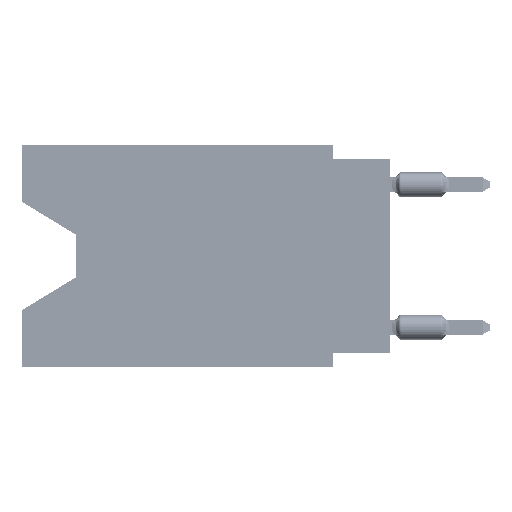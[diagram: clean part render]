
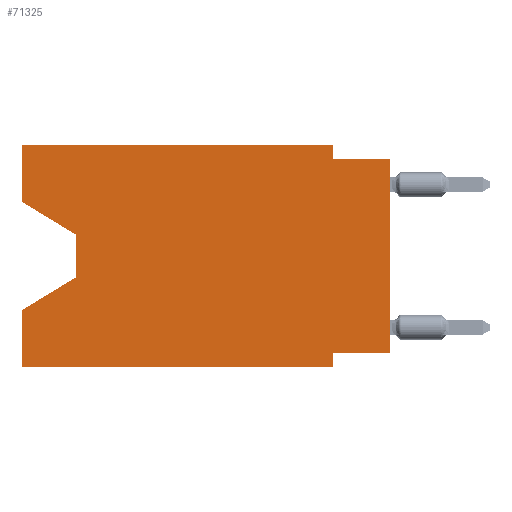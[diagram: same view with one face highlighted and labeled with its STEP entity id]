
A CAD part, left-side view. The second image highlights one B-rep face of the part: STEP entity #71325.
In plain terms, the highlighted planar face has unit normal (-1, 0, 0).
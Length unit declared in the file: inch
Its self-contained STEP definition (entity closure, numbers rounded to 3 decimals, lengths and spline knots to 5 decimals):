
#85 = CARTESIAN_POINT ( 'NONE',  ( 0., 0.645, 0. ) ) ;
#205 = CARTESIAN_POINT ( 'NONE',  ( 0., 0., 0. ) ) ;
#1108 = LINE ( 'NONE', #30797, #12926 ) ;
#4116 = EDGE_CURVE ( 'NONE', #9246, #67004, #49657, .T. ) ;
#4400 = EDGE_CURVE ( 'NONE', #48694, #24172, #54074, .T. ) ;
#4721 = ORIENTED_EDGE ( 'NONE', *, *, #23242, .F. ) ;
#5830 = CARTESIAN_POINT ( 'NONE',  ( 0., 0.645, -0.39 ) ) ;
#6450 = VECTOR ( 'NONE', #14433, 39.37008 ) ;
#6566 = VECTOR ( 'NONE', #40404, 39.37008 ) ;
#7133 = EDGE_CURVE ( 'NONE', #48694, #78525, #32270, .T. ) ;
#8567 = DIRECTION ( 'NONE',  ( 1., 0., 0. ) ) ;
#9246 = VERTEX_POINT ( 'NONE', #50335 ) ;
#9248 = LINE ( 'NONE', #72170, #31322 ) ;
#9652 = DIRECTION ( 'NONE',  ( 0., -0.855, -0.519 ) ) ;
#9934 = CARTESIAN_POINT ( 'NONE',  ( 0., 0.645, 0. ) ) ;
#10221 = CARTESIAN_POINT ( 'NONE',  ( 0., 0., -0.365 ) ) ;
#10315 = CARTESIAN_POINT ( 'NONE',  ( 0., 0.55, -0.158 ) ) ;
#10739 = VECTOR ( 'NONE', #42714, 39.37008 ) ;
#11453 = CARTESIAN_POINT ( 'NONE',  ( 0., 0.55, -0.158 ) ) ;
#12619 = ORIENTED_EDGE ( 'NONE', *, *, #4400, .F. ) ;
#12926 = VECTOR ( 'NONE', #68530, 39.37008 ) ;
#12966 = VERTEX_POINT ( 'NONE', #50551 ) ;
#13065 = EDGE_CURVE ( 'NONE', #71305, #78525, #18894, .T. ) ;
#14186 = ORIENTED_EDGE ( 'NONE', *, *, #52523, .T. ) ;
#14433 = DIRECTION ( 'NONE',  ( 0., 0., -1. ) ) ;
#15061 = ORIENTED_EDGE ( 'NONE', *, *, #55617, .T. ) ;
#16561 = VERTEX_POINT ( 'NONE', #10315 ) ;
#16594 = ORIENTED_EDGE ( 'NONE', *, *, #4116, .T. ) ;
#18894 = LINE ( 'NONE', #74912, #41798 ) ;
#19269 = DIRECTION ( 'NONE',  ( 0., 0., 1. ) ) ;
#19307 = VECTOR ( 'NONE', #73506, 39.37008 ) ;
#20121 = CARTESIAN_POINT ( 'NONE',  ( 0., 0.1, -0.39 ) ) ;
#21328 = CARTESIAN_POINT ( 'NONE',  ( 0., 0.1, -0.39 ) ) ;
#22410 = CARTESIAN_POINT ( 'NONE',  ( 0., 0.55, -0.232 ) ) ;
#22863 = CARTESIAN_POINT ( 'NONE',  ( 0., 0.645, -0.28975 ) ) ;
#23242 = EDGE_CURVE ( 'NONE', #24172, #67004, #46086, .T. ) ;
#24172 = VERTEX_POINT ( 'NONE', #58494 ) ;
#24850 = DIRECTION ( 'NONE',  ( 0., -1., 0. ) ) ;
#25305 = EDGE_CURVE ( 'NONE', #12966, #71305, #51599, .T. ) ;
#25319 = VECTOR ( 'NONE', #71940, 39.37008 ) ;
#29825 = VERTEX_POINT ( 'NONE', #40304 ) ;
#30617 = DIRECTION ( 'NONE',  ( 0., -1., 0. ) ) ;
#30797 = CARTESIAN_POINT ( 'NONE',  ( 0., 0.645, 0. ) ) ;
#31322 = VECTOR ( 'NONE', #9652, 39.37008 ) ;
#32270 = LINE ( 'NONE', #205, #74461 ) ;
#33681 = ORIENTED_EDGE ( 'NONE', *, *, #46680, .F. ) ;
#35033 = ORIENTED_EDGE ( 'NONE', *, *, #13065, .F. ) ;
#36433 = EDGE_CURVE ( 'NONE', #29825, #74711, #1108, .T. ) ;
#36576 = CARTESIAN_POINT ( 'NONE',  ( 0., 0.55, -0.232 ) ) ;
#37591 = CARTESIAN_POINT ( 'NONE',  ( 0., 0.645, 0. ) ) ;
#38622 = PLANE ( 'NONE',  #73836 ) ;
#39627 = VERTEX_POINT ( 'NONE', #22863 ) ;
#40304 = CARTESIAN_POINT ( 'NONE',  ( 0., 0.645, -0.10025 ) ) ;
#40404 = DIRECTION ( 'NONE',  ( 0., 0., 1. ) ) ;
#41792 = EDGE_CURVE ( 'NONE', #16561, #75496, #66691, .T. ) ;
#41798 = VECTOR ( 'NONE', #56646, 39.37008 ) ;
#42714 = DIRECTION ( 'NONE',  ( 0., 0., -1. ) ) ;
#44713 = FACE_OUTER_BOUND ( 'NONE', #45901, .T. ) ;
#45074 = VECTOR ( 'NONE', #24850, 39.37008 ) ;
#45112 = CARTESIAN_POINT ( 'NONE',  ( 0., 0.1, -0.025 ) ) ;
#45301 = ORIENTED_EDGE ( 'NONE', *, *, #36433, .F. ) ;
#45901 = EDGE_LOOP ( 'NONE', ( #15061, #56737, #14186, #62089, #16594, #4721, #12619, #48532, #35033, #59098, #33681, #45301 ) ) ;
#46086 = LINE ( 'NONE', #20121, #6450 ) ;
#46680 = EDGE_CURVE ( 'NONE', #74711, #12966, #55700, .T. ) ;
#48532 = ORIENTED_EDGE ( 'NONE', *, *, #7133, .T. ) ;
#48651 = VECTOR ( 'NONE', #64592, 39.37008 ) ;
#48694 = VERTEX_POINT ( 'NONE', #70020 ) ;
#49657 = LINE ( 'NONE', #5830, #57388 ) ;
#50335 = CARTESIAN_POINT ( 'NONE',  ( 0., 0.645, -0.39 ) ) ;
#50551 = CARTESIAN_POINT ( 'NONE',  ( 0., 0.1, 0. ) ) ;
#51599 = LINE ( 'NONE', #64190, #48651 ) ;
#52523 = EDGE_CURVE ( 'NONE', #75496, #39627, #66232, .T. ) ;
#54074 = LINE ( 'NONE', #10221, #25319 ) ;
#55617 = EDGE_CURVE ( 'NONE', #29825, #16561, #9248, .T. ) ;
#55700 = LINE ( 'NONE', #85, #45074 ) ;
#56646 = DIRECTION ( 'NONE',  ( 0., -1., 0. ) ) ;
#56737 = ORIENTED_EDGE ( 'NONE', *, *, #41792, .T. ) ;
#57388 = VECTOR ( 'NONE', #30617, 39.37008 ) ;
#58494 = CARTESIAN_POINT ( 'NONE',  ( 0., 0.1, -0.365 ) ) ;
#59098 = ORIENTED_EDGE ( 'NONE', *, *, #25305, .F. ) ;
#60950 = CARTESIAN_POINT ( 'NONE',  ( 0., 0., -0.025 ) ) ;
#61488 = EDGE_CURVE ( 'NONE', #9246, #39627, #78539, .T. ) ;
#62089 = ORIENTED_EDGE ( 'NONE', *, *, #61488, .F. ) ;
#63377 = DIRECTION ( 'NONE',  ( 0., 0., -1. ) ) ;
#64182 = CARTESIAN_POINT ( 'NONE',  ( 0., 0.645, 0. ) ) ;
#64190 = CARTESIAN_POINT ( 'NONE',  ( 0., 0.1, 0. ) ) ;
#64592 = DIRECTION ( 'NONE',  ( 0., 0., -1. ) ) ;
#66232 = LINE ( 'NONE', #36576, #19307 ) ;
#66691 = LINE ( 'NONE', #11453, #10739 ) ;
#67004 = VERTEX_POINT ( 'NONE', #21328 ) ;
#68530 = DIRECTION ( 'NONE',  ( 0., 0., 1. ) ) ;
#70020 = CARTESIAN_POINT ( 'NONE',  ( 0., 0., -0.365 ) ) ;
#71305 = VERTEX_POINT ( 'NONE', #45112 ) ;
#71325 = ADVANCED_FACE ( 'NONE', ( #44713 ), #38622, .F. ) ;
#71940 = DIRECTION ( 'NONE',  ( 0., 1., 0. ) ) ;
#72170 = CARTESIAN_POINT ( 'NONE',  ( 0., 0.645, -0.10025 ) ) ;
#73506 = DIRECTION ( 'NONE',  ( 0., 0.855, -0.519 ) ) ;
#73836 = AXIS2_PLACEMENT_3D ( 'NONE', #64182, #8567, #63377 ) ;
#74461 = VECTOR ( 'NONE', #19269, 39.37008 ) ;
#74711 = VERTEX_POINT ( 'NONE', #37591 ) ;
#74912 = CARTESIAN_POINT ( 'NONE',  ( 0., 0., -0.025 ) ) ;
#75496 = VERTEX_POINT ( 'NONE', #22410 ) ;
#78525 = VERTEX_POINT ( 'NONE', #60950 ) ;
#78539 = LINE ( 'NONE', #9934, #6566 ) ;
